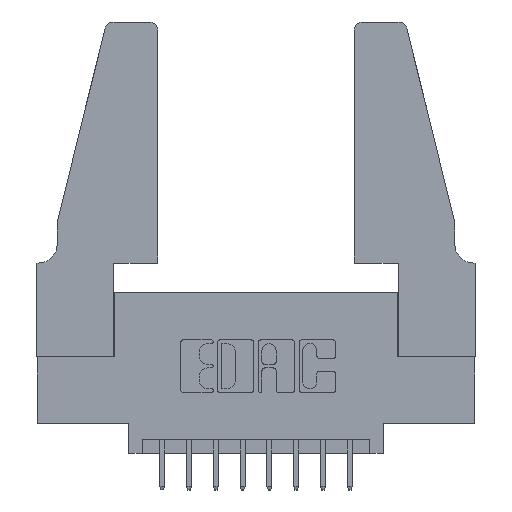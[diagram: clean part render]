
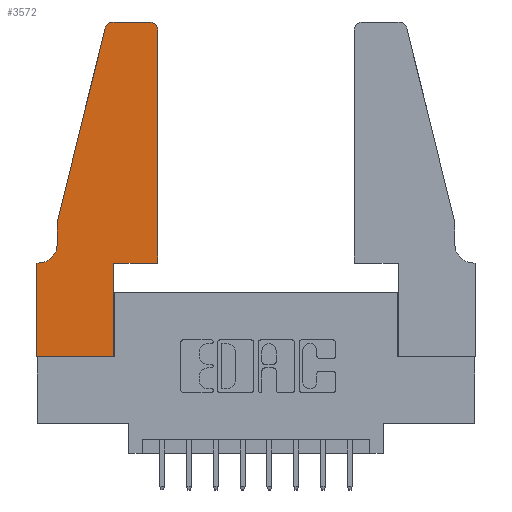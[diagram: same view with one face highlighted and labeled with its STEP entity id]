
A CAD part, top view. The second image highlights one B-rep face of the part: STEP entity #3572.
In plain terms, the highlighted planar face has unit normal (0, 0, 1).
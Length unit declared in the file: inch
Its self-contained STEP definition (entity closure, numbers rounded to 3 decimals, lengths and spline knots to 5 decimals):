
#11 = DIRECTION ( 'NONE',  ( 1., 0., 0. ) ) ;
#50 = CARTESIAN_POINT ( 'NONE',  ( 0.0755, 0.5, 0.37 ) ) ;
#257 = EDGE_CURVE ( 'NONE', #3150, #3783, #9765, .T. ) ;
#400 = VECTOR ( 'NONE', #7755, 39.37008 ) ;
#408 = EDGE_CURVE ( 'NONE', #3783, #5872, #11123, .T. ) ;
#435 = DIRECTION ( 'NONE',  ( -1., 0., 0. ) ) ;
#444 = EDGE_CURVE ( 'NONE', #2678, #9651, #4474, .T. ) ;
#560 = CARTESIAN_POINT ( 'NONE',  ( 0.0755, 0.35, 0.37 ) ) ;
#727 = CARTESIAN_POINT ( 'NONE',  ( 0.0055, 0.42, 0.37 ) ) ;
#861 = CARTESIAN_POINT ( 'NONE',  ( 0.4205, 1.22, 0.37 ) ) ;
#1008 = EDGE_CURVE ( 'NONE', #6414, #8407, #9580, .T. ) ;
#1484 = EDGE_CURVE ( 'NONE', #3100, #6414, #10628, .T. ) ;
#1502 = ORIENTED_EDGE ( 'NONE', *, *, #1484, .T. ) ;
#1786 = ORIENTED_EDGE ( 'NONE', *, *, #408, .T. ) ;
#1882 = DIRECTION ( 'NONE',  ( 0., 0., 1. ) ) ;
#1934 = LINE ( 'NONE', #50, #3823 ) ;
#2014 = EDGE_CURVE ( 'NONE', #5872, #3100, #1934, .T. ) ;
#2115 = ORIENTED_EDGE ( 'NONE', *, *, #3286, .T. ) ;
#2129 = CARTESIAN_POINT ( 'NONE',  ( 0., 0., 0.37 ) ) ;
#2146 = PLANE ( 'NONE',  #2627 ) ;
#2175 = VECTOR ( 'NONE', #8159, 39.37008 ) ;
#2188 = CARTESIAN_POINT ( 'NONE',  ( 0., 0., 0.37 ) ) ;
#2194 = VERTEX_POINT ( 'NONE', #13240 ) ;
#2289 = DIRECTION ( 'NONE',  ( 1., 0., 0. ) ) ;
#2336 = CARTESIAN_POINT ( 'NONE',  ( 0.25487, 1.22718, 0.37 ) ) ;
#2359 = VECTOR ( 'NONE', #8775, 39.37008 ) ;
#2433 = ORIENTED_EDGE ( 'NONE', *, *, #11090, .T. ) ;
#2627 = AXIS2_PLACEMENT_3D ( 'NONE', #7311, #12328, #7175 ) ;
#2678 = VERTEX_POINT ( 'NONE', #11448 ) ;
#2711 = VECTOR ( 'NONE', #435, 39.37008 ) ;
#2885 = CARTESIAN_POINT ( 'NONE',  ( 0.0055, 0.35, 0.37 ) ) ;
#2971 = ORIENTED_EDGE ( 'NONE', *, *, #3962, .T. ) ;
#2989 = VERTEX_POINT ( 'NONE', #2188 ) ;
#3033 = DIRECTION ( 'NONE',  ( -1., 0., 0. ) ) ;
#3100 = VERTEX_POINT ( 'NONE', #3740 ) ;
#3150 = VERTEX_POINT ( 'NONE', #10073 ) ;
#3174 = ORIENTED_EDGE ( 'NONE', *, *, #257, .T. ) ;
#3286 = EDGE_CURVE ( 'NONE', #9651, #4758, #12602, .T. ) ;
#3302 = VECTOR ( 'NONE', #7576, 39.37008 ) ;
#3421 = EDGE_CURVE ( 'NONE', #2989, #2678, #7388, .T. ) ;
#3572 = ADVANCED_FACE ( 'NONE', ( #3970 ), #2146, .T. ) ;
#3652 = LINE ( 'NONE', #4098, #8659 ) ;
#3685 = CARTESIAN_POINT ( 'NONE',  ( 0.2865, 0.35, 0.37 ) ) ;
#3740 = CARTESIAN_POINT ( 'NONE',  ( 0.0755, 0.42, 0.37 ) ) ;
#3746 = DIRECTION ( 'NONE',  ( 1., 0., 0. ) ) ;
#3783 = VERTEX_POINT ( 'NONE', #2336 ) ;
#3816 = ORIENTED_EDGE ( 'NONE', *, *, #1008, .T. ) ;
#3823 = VECTOR ( 'NONE', #6134, 39.37008 ) ;
#3962 = EDGE_CURVE ( 'NONE', #5213, #2194, #7184, .T. ) ;
#3970 = FACE_OUTER_BOUND ( 'NONE', #9331, .T. ) ;
#4098 = CARTESIAN_POINT ( 'NONE',  ( 0.2605, 1.25, 0.37 ) ) ;
#4163 = CARTESIAN_POINT ( 'NONE',  ( 0.0755, 0.5, 0.37 ) ) ;
#4179 = AXIS2_PLACEMENT_3D ( 'NONE', #861, #1882, #11 ) ;
#4444 = VECTOR ( 'NONE', #11326, 39.37008 ) ;
#4474 = LINE ( 'NONE', #8566, #400 ) ;
#4758 = VERTEX_POINT ( 'NONE', #8491 ) ;
#4915 = EDGE_CURVE ( 'NONE', #4758, #5213, #13003, .T. ) ;
#5213 = VERTEX_POINT ( 'NONE', #12722 ) ;
#5624 = EDGE_CURVE ( 'NONE', #8407, #2989, #9211, .T. ) ;
#5728 = ORIENTED_EDGE ( 'NONE', *, *, #3421, .T. ) ;
#5872 = VERTEX_POINT ( 'NONE', #12970 ) ;
#6004 = CARTESIAN_POINT ( 'NONE',  ( 0., 0.35, 0.37 ) ) ;
#6066 = CARTESIAN_POINT ( 'NONE',  ( 0.284, 1.22, 0.37 ) ) ;
#6134 = DIRECTION ( 'NONE',  ( 0., -1., 0. ) ) ;
#6221 = ORIENTED_EDGE ( 'NONE', *, *, #4915, .T. ) ;
#6414 = VERTEX_POINT ( 'NONE', #2885 ) ;
#6487 = VECTOR ( 'NONE', #2289, 39.37008 ) ;
#6924 = ORIENTED_EDGE ( 'NONE', *, *, #444, .T. ) ;
#7175 = DIRECTION ( 'NONE',  ( 1., 0., 0. ) ) ;
#7184 = CIRCLE ( 'NONE', #4179, 0.03 ) ;
#7311 = CARTESIAN_POINT ( 'NONE',  ( 0., 0.35, 0.37 ) ) ;
#7388 = LINE ( 'NONE', #11456, #6487 ) ;
#7576 = DIRECTION ( 'NONE',  ( 1., 0., 0. ) ) ;
#7755 = DIRECTION ( 'NONE',  ( 0., 1., 0. ) ) ;
#8105 = ORIENTED_EDGE ( 'NONE', *, *, #2014, .T. ) ;
#8159 = DIRECTION ( 'NONE',  ( 0., -1., 0. ) ) ;
#8407 = VERTEX_POINT ( 'NONE', #6004 ) ;
#8491 = CARTESIAN_POINT ( 'NONE',  ( 0.4505, 0.35, 0.37 ) ) ;
#8566 = CARTESIAN_POINT ( 'NONE',  ( 0.2865, 0.35, 0.37 ) ) ;
#8659 = VECTOR ( 'NONE', #3033, 39.37008 ) ;
#8775 = DIRECTION ( 'NONE',  ( 0., 1., 0. ) ) ;
#9144 = AXIS2_PLACEMENT_3D ( 'NONE', #727, #12993, #10969 ) ;
#9211 = LINE ( 'NONE', #2129, #2175 ) ;
#9331 = EDGE_LOOP ( 'NONE', ( #2433, #3174, #1786, #8105, #1502, #3816, #10983, #5728, #6924, #2115, #6221, #2971 ) ) ;
#9580 = LINE ( 'NONE', #560, #2711 ) ;
#9651 = VERTEX_POINT ( 'NONE', #3685 ) ;
#9765 = CIRCLE ( 'NONE', #11296, 0.03 ) ;
#9817 = CARTESIAN_POINT ( 'NONE',  ( 0.4505, 0.35, 0.37 ) ) ;
#10073 = CARTESIAN_POINT ( 'NONE',  ( 0.284, 1.25, 0.37 ) ) ;
#10628 = CIRCLE ( 'NONE', #9144, 0.07 ) ;
#10969 = DIRECTION ( 'NONE',  ( -1., 0., 0. ) ) ;
#10983 = ORIENTED_EDGE ( 'NONE', *, *, #5624, .T. ) ;
#11090 = EDGE_CURVE ( 'NONE', #2194, #3150, #3652, .T. ) ;
#11123 = LINE ( 'NONE', #4163, #4444 ) ;
#11296 = AXIS2_PLACEMENT_3D ( 'NONE', #6066, #12899, #3746 ) ;
#11326 = DIRECTION ( 'NONE',  ( -0.239, -0.971, 0. ) ) ;
#11448 = CARTESIAN_POINT ( 'NONE',  ( 0.2865, 0., 0.37 ) ) ;
#11456 = CARTESIAN_POINT ( 'NONE',  ( 0., 0., 0.37 ) ) ;
#11712 = CARTESIAN_POINT ( 'NONE',  ( 0.4505, 0.35, 0.37 ) ) ;
#12328 = DIRECTION ( 'NONE',  ( 0., 0., 1. ) ) ;
#12602 = LINE ( 'NONE', #11712, #3302 ) ;
#12722 = CARTESIAN_POINT ( 'NONE',  ( 0.4505, 1.22, 0.37 ) ) ;
#12899 = DIRECTION ( 'NONE',  ( 0., 0., 1. ) ) ;
#12970 = CARTESIAN_POINT ( 'NONE',  ( 0.0755, 0.5, 0.37 ) ) ;
#12993 = DIRECTION ( 'NONE',  ( 0., 0., -1. ) ) ;
#13003 = LINE ( 'NONE', #9817, #2359 ) ;
#13240 = CARTESIAN_POINT ( 'NONE',  ( 0.4205, 1.25, 0.37 ) ) ;
